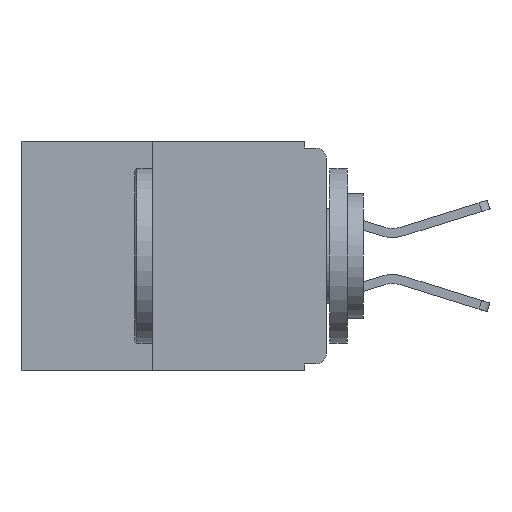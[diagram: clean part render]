
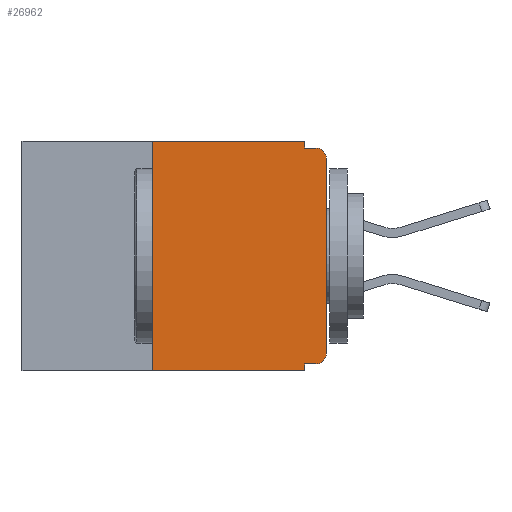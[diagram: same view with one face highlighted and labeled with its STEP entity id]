
A CAD part, left-side view. The second image highlights one B-rep face of the part: STEP entity #26962.
In plain terms, the highlighted planar face has unit normal (-1, 0, 0).
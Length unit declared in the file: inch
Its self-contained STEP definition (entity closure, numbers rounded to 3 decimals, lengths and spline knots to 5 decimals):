
#427 = AXIS2_PLACEMENT_3D ( 'NONE', #18492, #4955, #20769 ) ;
#727 = VERTEX_POINT ( 'NONE', #17143 ) ;
#913 = AXIS2_PLACEMENT_3D ( 'NONE', #5433, #21218, #7727 ) ;
#1675 = ORIENTED_EDGE ( 'NONE', *, *, #26247, .F. ) ;
#2258 = CARTESIAN_POINT ( 'NONE',  ( 0., 0.031, -0.33 ) ) ;
#2675 = ORIENTED_EDGE ( 'NONE', *, *, #7935, .F. ) ;
#2740 = ORIENTED_EDGE ( 'NONE', *, *, #28882, .F. ) ;
#2931 = CARTESIAN_POINT ( 'NONE',  ( 0., 0., -0.025 ) ) ;
#3530 = LINE ( 'NONE', #5778, #26191 ) ;
#4607 = AXIS2_PLACEMENT_3D ( 'NONE', #8270, #24030, #10546 ) ;
#4955 = DIRECTION ( 'NONE',  ( -1., 0., 0. ) ) ;
#5433 = CARTESIAN_POINT ( 'NONE',  ( 0., 0.437, 0. ) ) ;
#5778 = CARTESIAN_POINT ( 'NONE',  ( 0., 0., -0.32 ) ) ;
#5852 = LINE ( 'NONE', #16443, #29133 ) ;
#6053 = LINE ( 'NONE', #24756, #29306 ) ;
#6151 = CARTESIAN_POINT ( 'NONE',  ( 0., 0.031, 0. ) ) ;
#6783 = VERTEX_POINT ( 'NONE', #14258 ) ;
#6830 = VECTOR ( 'NONE', #8406, 39.37008 ) ;
#6838 = VECTOR ( 'NONE', #16359, 39.37008 ) ;
#7032 = VERTEX_POINT ( 'NONE', #8220 ) ;
#7300 = DIRECTION ( 'NONE',  ( 0., -1., 0. ) ) ;
#7727 = DIRECTION ( 'NONE',  ( 0., 0., -1. ) ) ;
#7887 = LINE ( 'NONE', #18525, #25167 ) ;
#7935 = EDGE_CURVE ( 'NONE', #8028, #12786, #7887, .T. ) ;
#8015 = VERTEX_POINT ( 'NONE', #2931 ) ;
#8028 = VERTEX_POINT ( 'NONE', #18910 ) ;
#8220 = CARTESIAN_POINT ( 'NONE',  ( 0., 0., -0.305 ) ) ;
#8270 = CARTESIAN_POINT ( 'NONE',  ( 0., 0.015, -0.305 ) ) ;
#8406 = DIRECTION ( 'NONE',  ( 0., 0., -1. ) ) ;
#8482 = CIRCLE ( 'NONE', #4607, 0.015 ) ;
#8939 = ORIENTED_EDGE ( 'NONE', *, *, #16076, .T. ) ;
#8999 = VERTEX_POINT ( 'NONE', #29111 ) ;
#9105 = VECTOR ( 'NONE', #11425, 39.37008 ) ;
#9380 = CARTESIAN_POINT ( 'NONE',  ( 0., 0.25, -0.33 ) ) ;
#10312 = DIRECTION ( 'NONE',  ( 0., 1., 0. ) ) ;
#10546 = DIRECTION ( 'NONE',  ( 0., 0., -1. ) ) ;
#10597 = ORIENTED_EDGE ( 'NONE', *, *, #20040, .T. ) ;
#11425 = DIRECTION ( 'NONE',  ( 0., -1., 0. ) ) ;
#12121 = LINE ( 'NONE', #18610, #6838 ) ;
#12786 = VERTEX_POINT ( 'NONE', #27649 ) ;
#12961 = VERTEX_POINT ( 'NONE', #28244 ) ;
#13541 = LINE ( 'NONE', #6151, #6830 ) ;
#14184 = DIRECTION ( 'NONE',  ( 0., -1., 0. ) ) ;
#14258 = CARTESIAN_POINT ( 'NONE',  ( 0., 0.031, -0.32 ) ) ;
#14452 = PLANE ( 'NONE',  #913 ) ;
#15813 = DIRECTION ( 'NONE',  ( 0., 0., -1. ) ) ;
#15884 = CARTESIAN_POINT ( 'NONE',  ( 0., 0.437, -0.33 ) ) ;
#16076 = EDGE_CURVE ( 'NONE', #8999, #7032, #8482, .T. ) ;
#16359 = DIRECTION ( 'NONE',  ( 0., 0., 1. ) ) ;
#16443 = CARTESIAN_POINT ( 'NONE',  ( 0., 0.437, 0. ) ) ;
#16978 = VERTEX_POINT ( 'NONE', #2258 ) ;
#17143 = CARTESIAN_POINT ( 'NONE',  ( 0., 0.25, -0.33 ) ) ;
#17374 = ORIENTED_EDGE ( 'NONE', *, *, #24343, .T. ) ;
#18492 = CARTESIAN_POINT ( 'NONE',  ( 0., 0.015, -0.025 ) ) ;
#18525 = CARTESIAN_POINT ( 'NONE',  ( 0., 0., -0.01 ) ) ;
#18610 = CARTESIAN_POINT ( 'NONE',  ( 0., 0., 0. ) ) ;
#18822 = LINE ( 'NONE', #9380, #29394 ) ;
#18910 = CARTESIAN_POINT ( 'NONE',  ( 0., 0.031, -0.01 ) ) ;
#20040 = EDGE_CURVE ( 'NONE', #7032, #8015, #12121, .T. ) ;
#20719 = ORIENTED_EDGE ( 'NONE', *, *, #28157, .F. ) ;
#20769 = DIRECTION ( 'NONE',  ( 0., 0., -1. ) ) ;
#20895 = CARTESIAN_POINT ( 'NONE',  ( 0., 0.031, 0. ) ) ;
#21188 = ORIENTED_EDGE ( 'NONE', *, *, #27373, .F. ) ;
#21218 = DIRECTION ( 'NONE',  ( 1., 0., 0. ) ) ;
#21416 = ORIENTED_EDGE ( 'NONE', *, *, #23588, .T. ) ;
#21793 = LINE ( 'NONE', #15884, #9105 ) ;
#22731 = FACE_OUTER_BOUND ( 'NONE', #26178, .T. ) ;
#22817 = EDGE_CURVE ( 'NONE', #6783, #16978, #6053, .T. ) ;
#23587 = CIRCLE ( 'NONE', #427, 0.015 ) ;
#23588 = EDGE_CURVE ( 'NONE', #8015, #12786, #23587, .T. ) ;
#24030 = DIRECTION ( 'NONE',  ( -1., 0., 0. ) ) ;
#24343 = EDGE_CURVE ( 'NONE', #727, #16978, #21793, .T. ) ;
#24756 = CARTESIAN_POINT ( 'NONE',  ( 0., 0.031, -0.33 ) ) ;
#25167 = VECTOR ( 'NONE', #7300, 39.37008 ) ;
#26178 = EDGE_LOOP ( 'NONE', ( #10597, #21416, #2675, #2740, #1675, #21188, #17374, #27651, #20719, #8939 ) ) ;
#26191 = VECTOR ( 'NONE', #10312, 39.37008 ) ;
#26247 = EDGE_CURVE ( 'NONE', #12961, #27448, #5852, .T. ) ;
#26962 = ADVANCED_FACE ( 'NONE', ( #22731 ), #14452, .F. ) ;
#27373 = EDGE_CURVE ( 'NONE', #727, #12961, #18822, .T. ) ;
#27421 = DIRECTION ( 'NONE',  ( 0., 0., 1. ) ) ;
#27448 = VERTEX_POINT ( 'NONE', #20895 ) ;
#27649 = CARTESIAN_POINT ( 'NONE',  ( 0., 0.015, -0.01 ) ) ;
#27651 = ORIENTED_EDGE ( 'NONE', *, *, #22817, .F. ) ;
#28157 = EDGE_CURVE ( 'NONE', #8999, #6783, #3530, .T. ) ;
#28244 = CARTESIAN_POINT ( 'NONE',  ( 0., 0.25, 0. ) ) ;
#28882 = EDGE_CURVE ( 'NONE', #27448, #8028, #13541, .T. ) ;
#29111 = CARTESIAN_POINT ( 'NONE',  ( 0., 0.015, -0.32 ) ) ;
#29133 = VECTOR ( 'NONE', #14184, 39.37008 ) ;
#29306 = VECTOR ( 'NONE', #15813, 39.37008 ) ;
#29394 = VECTOR ( 'NONE', #27421, 39.37008 ) ;
